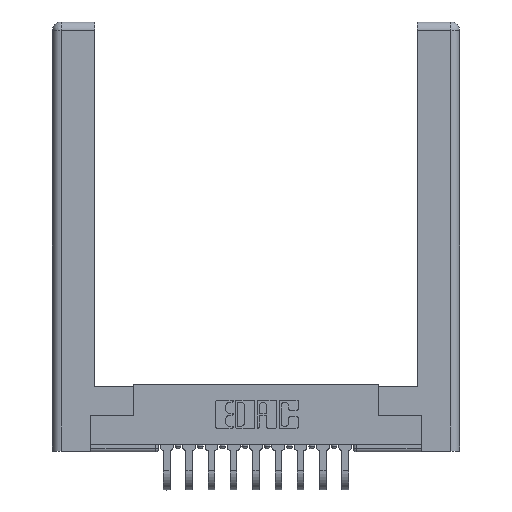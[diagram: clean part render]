
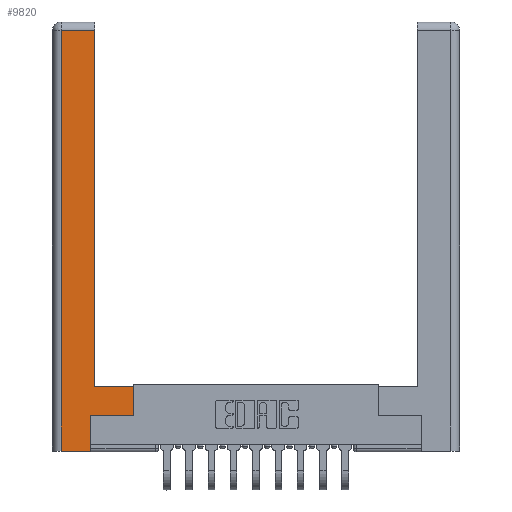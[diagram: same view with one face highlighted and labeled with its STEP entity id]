
A CAD part, top view. The second image highlights one B-rep face of the part: STEP entity #9820.
In plain terms, the highlighted planar face has unit normal (0, 0, 1).
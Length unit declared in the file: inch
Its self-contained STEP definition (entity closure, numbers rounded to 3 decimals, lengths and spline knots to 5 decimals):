
#152 = CARTESIAN_POINT ( 'NONE',  ( 0.265, 0., 0. ) ) ;
#231 = EDGE_CURVE ( 'NONE', #4799, #11607, #10400, .T. ) ;
#330 = CARTESIAN_POINT ( 'NONE',  ( 0.0615, 2.94, 0. ) ) ;
#352 = DIRECTION ( 'NONE',  ( 0., 1., 0. ) ) ;
#879 = VECTOR ( 'NONE', #13585, 39.37008 ) ;
#924 = ORIENTED_EDGE ( 'NONE', *, *, #11937, .T. ) ;
#1022 = CARTESIAN_POINT ( 'NONE',  ( 0.295, 0.45, 0. ) ) ;
#1660 = CARTESIAN_POINT ( 'NONE',  ( 0.0615, 0., 0. ) ) ;
#2100 = CARTESIAN_POINT ( 'NONE',  ( 0.265, 0.245, 0. ) ) ;
#2497 = EDGE_CURVE ( 'NONE', #6276, #12510, #5062, .T. ) ;
#2601 = DIRECTION ( 'NONE',  ( 1., 0., 0. ) ) ;
#2610 = VERTEX_POINT ( 'NONE', #14211 ) ;
#2901 = LINE ( 'NONE', #1660, #11952 ) ;
#3334 = FACE_OUTER_BOUND ( 'NONE', #8373, .T. ) ;
#3616 = EDGE_CURVE ( 'NONE', #12510, #4327, #13877, .T. ) ;
#3906 = EDGE_CURVE ( 'NONE', #9999, #6276, #8404, .T. ) ;
#3969 = CARTESIAN_POINT ( 'NONE',  ( 0.295, 0.45, 0. ) ) ;
#4020 = VECTOR ( 'NONE', #2601, 39.37008 ) ;
#4162 = DIRECTION ( 'NONE',  ( 0., 1., 0. ) ) ;
#4216 = DIRECTION ( 'NONE',  ( -1., 0., 0. ) ) ;
#4327 = VERTEX_POINT ( 'NONE', #5073 ) ;
#4507 = CARTESIAN_POINT ( 'NONE',  ( 0., 0., 0. ) ) ;
#4597 = CARTESIAN_POINT ( 'NONE',  ( 0.565, 0.245, 0. ) ) ;
#4799 = VERTEX_POINT ( 'NONE', #14363 ) ;
#4807 = DIRECTION ( 'NONE',  ( -1., 0., 0. ) ) ;
#5062 = LINE ( 'NONE', #9549, #4020 ) ;
#5073 = CARTESIAN_POINT ( 'NONE',  ( 0.565, 0.45, 0. ) ) ;
#5302 = VECTOR ( 'NONE', #8479, 39.37008 ) ;
#5434 = CARTESIAN_POINT ( 'NONE',  ( 0.0615, 2.94, 0. ) ) ;
#5631 = ORIENTED_EDGE ( 'NONE', *, *, #3906, .T. ) ;
#5973 = DIRECTION ( 'NONE',  ( 0., -1., 0. ) ) ;
#6022 = ORIENTED_EDGE ( 'NONE', *, *, #12733, .T. ) ;
#6276 = VERTEX_POINT ( 'NONE', #8919 ) ;
#6669 = CARTESIAN_POINT ( 'NONE',  ( 0.265, 0., 0. ) ) ;
#6720 = AXIS2_PLACEMENT_3D ( 'NONE', #4507, #12142, #4216 ) ;
#6846 = ORIENTED_EDGE ( 'NONE', *, *, #3616, .T. ) ;
#6985 = EDGE_CURVE ( 'NONE', #2610, #9999, #13511, .T. ) ;
#7304 = VECTOR ( 'NONE', #352, 39.37008 ) ;
#7375 = DIRECTION ( 'NONE',  ( -1., 0., 0. ) ) ;
#8083 = ORIENTED_EDGE ( 'NONE', *, *, #231, .T. ) ;
#8373 = EDGE_LOOP ( 'NONE', ( #11456, #8083, #6022, #14108, #5631, #12745, #6846, #924 ) ) ;
#8404 = LINE ( 'NONE', #2100, #10846 ) ;
#8479 = DIRECTION ( 'NONE',  ( 0., 1., 0. ) ) ;
#8692 = LINE ( 'NONE', #14368, #5302 ) ;
#8792 = EDGE_CURVE ( 'NONE', #14414, #4799, #8692, .T. ) ;
#8919 = CARTESIAN_POINT ( 'NONE',  ( 0.265, 0.245, 0. ) ) ;
#9549 = CARTESIAN_POINT ( 'NONE',  ( 0.565, 0.245, 0. ) ) ;
#9820 = ADVANCED_FACE ( 'NONE', ( #3334 ), #9927, .F. ) ;
#9927 = PLANE ( 'NONE',  #6720 ) ;
#9999 = VERTEX_POINT ( 'NONE', #152 ) ;
#10400 = LINE ( 'NONE', #330, #11957 ) ;
#10846 = VECTOR ( 'NONE', #4162, 39.37008 ) ;
#11456 = ORIENTED_EDGE ( 'NONE', *, *, #8792, .T. ) ;
#11607 = VERTEX_POINT ( 'NONE', #5434 ) ;
#11665 = CARTESIAN_POINT ( 'NONE',  ( 0.565, 0.45, 0. ) ) ;
#11719 = VECTOR ( 'NONE', #7375, 39.37008 ) ;
#11937 = EDGE_CURVE ( 'NONE', #4327, #14414, #14031, .T. ) ;
#11952 = VECTOR ( 'NONE', #5973, 39.37008 ) ;
#11957 = VECTOR ( 'NONE', #4807, 39.37008 ) ;
#12142 = DIRECTION ( 'NONE',  ( 0., 0., -1. ) ) ;
#12510 = VERTEX_POINT ( 'NONE', #4597 ) ;
#12733 = EDGE_CURVE ( 'NONE', #11607, #2610, #2901, .T. ) ;
#12745 = ORIENTED_EDGE ( 'NONE', *, *, #2497, .T. ) ;
#13511 = LINE ( 'NONE', #6669, #879 ) ;
#13585 = DIRECTION ( 'NONE',  ( 1., 0., 0. ) ) ;
#13877 = LINE ( 'NONE', #11665, #7304 ) ;
#14031 = LINE ( 'NONE', #3969, #11719 ) ;
#14108 = ORIENTED_EDGE ( 'NONE', *, *, #6985, .T. ) ;
#14211 = CARTESIAN_POINT ( 'NONE',  ( 0.0615, 0., 0. ) ) ;
#14363 = CARTESIAN_POINT ( 'NONE',  ( 0.295, 2.94, 0. ) ) ;
#14368 = CARTESIAN_POINT ( 'NONE',  ( 0.295, 3., 0. ) ) ;
#14414 = VERTEX_POINT ( 'NONE', #1022 ) ;
